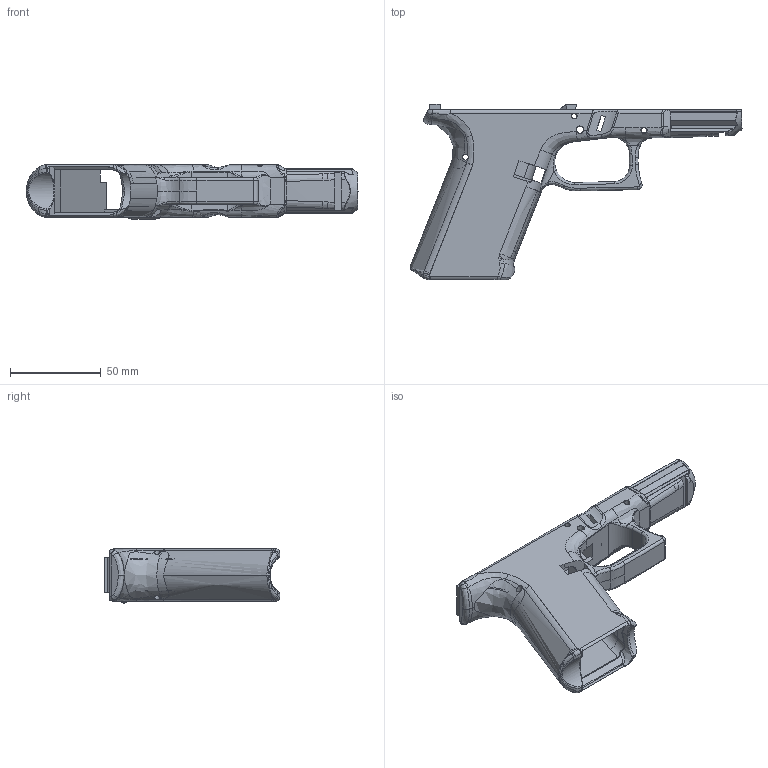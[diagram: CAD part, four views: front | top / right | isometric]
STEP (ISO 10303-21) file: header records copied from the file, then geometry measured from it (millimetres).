
FILE_DESCRIPTION(/* description */ (''),/* implementation_level */ '2;1');
FILE_NAME(/* name */ 'FMDA DD19.2 V1.2 G5Spring Frame.stp',/* time_stamp */ '2021-02-04T13:51:00-06:00',/* author */ ('johne'),/* organization */ (''),/* preprocessor_version */ 'ST-DEVELOPER v18',/* originating_system */ 'Autodesk Inventor 2020',/* authorisation */ '');
FILE_SCHEMA (('AUTOMOTIVE_DESIGN { 1 0 10303 214 3 1 1 }'));
Products named in the file (1): FMDA G19.2 V1.2 G5 Spring
Bounding box: 183.22 x 97 x 29.84 mm (x, y, z)
Volume: 78212.5 mm3; surface area: 43433 mm2
Topology: 1 solids, 3 shells, 669 faces, 1929 edges, 1234 vertices
Faces by surface type: bspline 292, plane 189, cylinder 133, torus 29, sphere 14, cone 12
Full cylindrical faces by diameter (mm): 2 x1, 3 x4, 3.2 x2, 3.81 x1, 4 x2
Entity records: 53914 total; most frequent: CARTESIAN_POINT 37608, ORIENTED_EDGE 3838, DIRECTION 2576, EDGE_CURVE 1919, VERTEX_POINT 1237, AXIS2_PLACEMENT_3D 946, LINE 684, VECTOR 684
